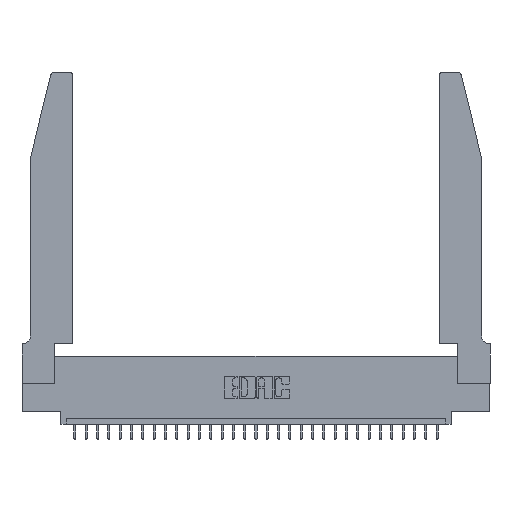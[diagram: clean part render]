
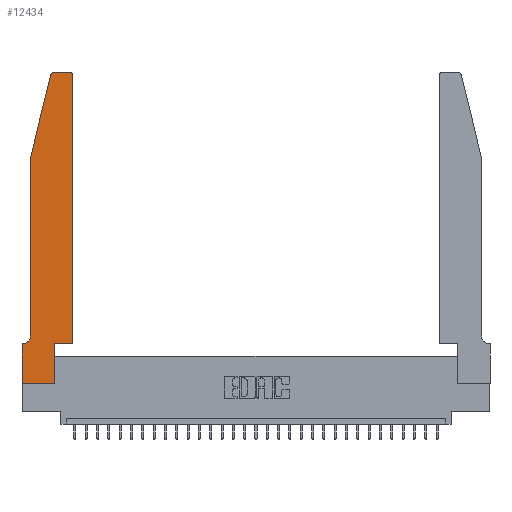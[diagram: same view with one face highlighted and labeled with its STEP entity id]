
A CAD part, top view. The second image highlights one B-rep face of the part: STEP entity #12434.
In plain terms, the highlighted planar face has unit normal (0, 0, 1).
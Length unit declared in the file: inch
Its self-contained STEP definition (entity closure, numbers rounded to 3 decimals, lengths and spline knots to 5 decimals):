
#24 = CARTESIAN_POINT ( 'NONE',  ( 0.4505, 0.35, 0.37 ) ) ;
#184 = DIRECTION ( 'NONE',  ( 0., 1., 0. ) ) ;
#619 = DIRECTION ( 'NONE',  ( -1., 0., 0. ) ) ;
#630 = VERTEX_POINT ( 'NONE', #18062 ) ;
#817 = LINE ( 'NONE', #17613, #28655 ) ;
#1134 = DIRECTION ( 'NONE',  ( 1., 0., 0. ) ) ;
#1655 = DIRECTION ( 'NONE',  ( -0.239, -0.971, 0. ) ) ;
#1787 = ORIENTED_EDGE ( 'NONE', *, *, #20117, .T. ) ;
#1981 = AXIS2_PLACEMENT_3D ( 'NONE', #28719, #7492, #7812 ) ;
#2095 = ORIENTED_EDGE ( 'NONE', *, *, #12523, .T. ) ;
#2313 = CARTESIAN_POINT ( 'NONE',  ( 0., 0., 0.37 ) ) ;
#2774 = CIRCLE ( 'NONE', #6782, 0.03 ) ;
#2963 = DIRECTION ( 'NONE',  ( 0., -1., 0. ) ) ;
#3488 = VERTEX_POINT ( 'NONE', #30178 ) ;
#3689 = EDGE_CURVE ( 'NONE', #6825, #12220, #12042, .T. ) ;
#4050 = EDGE_CURVE ( 'NONE', #20347, #630, #19760, .T. ) ;
#4278 = DIRECTION ( 'NONE',  ( 0., 0., -1. ) ) ;
#4942 = VERTEX_POINT ( 'NONE', #12701 ) ;
#6218 = AXIS2_PLACEMENT_3D ( 'NONE', #19846, #10734, #8375 ) ;
#6300 = ORIENTED_EDGE ( 'NONE', *, *, #28760, .T. ) ;
#6625 = CARTESIAN_POINT ( 'NONE',  ( 0.0055, 0.35, 0.37 ) ) ;
#6782 = AXIS2_PLACEMENT_3D ( 'NONE', #7217, #21823, #21666 ) ;
#6825 = VERTEX_POINT ( 'NONE', #28835 ) ;
#7217 = CARTESIAN_POINT ( 'NONE',  ( 0.4205, 2.72, 0.37 ) ) ;
#7363 = ORIENTED_EDGE ( 'NONE', *, *, #13226, .T. ) ;
#7492 = DIRECTION ( 'NONE',  ( 0., 0., 1. ) ) ;
#7812 = DIRECTION ( 'NONE',  ( 1., 0., 0. ) ) ;
#8301 = LINE ( 'NONE', #17561, #20855 ) ;
#8375 = DIRECTION ( 'NONE',  ( 1., 0., 0. ) ) ;
#9555 = FACE_OUTER_BOUND ( 'NONE', #12694, .T. ) ;
#9701 = ORIENTED_EDGE ( 'NONE', *, *, #3689, .T. ) ;
#10126 = LINE ( 'NONE', #10582, #14154 ) ;
#10496 = CARTESIAN_POINT ( 'NONE',  ( 0.0755, 0.35, 0.37 ) ) ;
#10582 = CARTESIAN_POINT ( 'NONE',  ( 0.2605, 2.75, 0.37 ) ) ;
#10734 = DIRECTION ( 'NONE',  ( 0., 0., 1. ) ) ;
#11142 = VERTEX_POINT ( 'NONE', #6625 ) ;
#11200 = CARTESIAN_POINT ( 'NONE',  ( 0.0055, 0.42, 0.37 ) ) ;
#12042 = LINE ( 'NONE', #2313, #20782 ) ;
#12220 = VERTEX_POINT ( 'NONE', #27486 ) ;
#12434 = ADVANCED_FACE ( 'NONE', ( #9555 ), #19130, .T. ) ;
#12523 = EDGE_CURVE ( 'NONE', #12220, #22360, #26992, .T. ) ;
#12694 = EDGE_LOOP ( 'NONE', ( #1787, #26218, #27043, #19061, #6300, #14378, #14070, #9701, #2095, #24430, #7363, #16059 ) ) ;
#12701 = CARTESIAN_POINT ( 'NONE',  ( 0.4505, 2.72, 0.37 ) ) ;
#12986 = VECTOR ( 'NONE', #1655, 39.37008 ) ;
#13226 = EDGE_CURVE ( 'NONE', #3488, #4942, #14142, .T. ) ;
#13832 = VERTEX_POINT ( 'NONE', #27920 ) ;
#14070 = ORIENTED_EDGE ( 'NONE', *, *, #25275, .T. ) ;
#14142 = LINE ( 'NONE', #24, #26100 ) ;
#14154 = VECTOR ( 'NONE', #29294, 39.37008 ) ;
#14342 = EDGE_CURVE ( 'NONE', #630, #13832, #19048, .T. ) ;
#14378 = ORIENTED_EDGE ( 'NONE', *, *, #29423, .T. ) ;
#14884 = DIRECTION ( 'NONE',  ( 0., 1., 0. ) ) ;
#15767 = VERTEX_POINT ( 'NONE', #30787 ) ;
#15843 = CARTESIAN_POINT ( 'NONE',  ( 0.0755, 2., 0.37 ) ) ;
#16059 = ORIENTED_EDGE ( 'NONE', *, *, #25061, .T. ) ;
#16525 = CARTESIAN_POINT ( 'NONE',  ( 0.0755, 2., 0.37 ) ) ;
#16922 = CARTESIAN_POINT ( 'NONE',  ( 0.2865, 0.35, 0.37 ) ) ;
#17038 = VECTOR ( 'NONE', #14884, 39.37008 ) ;
#17561 = CARTESIAN_POINT ( 'NONE',  ( 0., 0., 0.37 ) ) ;
#17613 = CARTESIAN_POINT ( 'NONE',  ( 0.4505, 0.35, 0.37 ) ) ;
#18062 = CARTESIAN_POINT ( 'NONE',  ( 0.25487, 2.72718, 0.37 ) ) ;
#18419 = DIRECTION ( 'NONE',  ( -1., 0., 0. ) ) ;
#18483 = EDGE_CURVE ( 'NONE', #22360, #3488, #817, .T. ) ;
#19048 = LINE ( 'NONE', #16525, #12986 ) ;
#19061 = ORIENTED_EDGE ( 'NONE', *, *, #29524, .T. ) ;
#19130 = PLANE ( 'NONE',  #1981 ) ;
#19277 = DIRECTION ( 'NONE',  ( 1., 0., 0. ) ) ;
#19760 = CIRCLE ( 'NONE', #6218, 0.03 ) ;
#19846 = CARTESIAN_POINT ( 'NONE',  ( 0.284, 2.72, 0.37 ) ) ;
#20117 = EDGE_CURVE ( 'NONE', #29048, #20347, #10126, .T. ) ;
#20347 = VERTEX_POINT ( 'NONE', #26129 ) ;
#20603 = VECTOR ( 'NONE', #22918, 39.37008 ) ;
#20782 = VECTOR ( 'NONE', #19277, 39.37008 ) ;
#20855 = VECTOR ( 'NONE', #2963, 39.37008 ) ;
#21666 = DIRECTION ( 'NONE',  ( 1., 0., 0. ) ) ;
#21823 = DIRECTION ( 'NONE',  ( 0., 0., 1. ) ) ;
#22360 = VERTEX_POINT ( 'NONE', #26810 ) ;
#22918 = DIRECTION ( 'NONE',  ( 0., -1., 0. ) ) ;
#24430 = ORIENTED_EDGE ( 'NONE', *, *, #18483, .T. ) ;
#24562 = AXIS2_PLACEMENT_3D ( 'NONE', #11200, #4278, #18419 ) ;
#24852 = CARTESIAN_POINT ( 'NONE',  ( 0.4205, 2.75, 0.37 ) ) ;
#25061 = EDGE_CURVE ( 'NONE', #4942, #29048, #2774, .T. ) ;
#25275 = EDGE_CURVE ( 'NONE', #15767, #6825, #8301, .T. ) ;
#25448 = CARTESIAN_POINT ( 'NONE',  ( 0.0755, 0.42, 0.37 ) ) ;
#26100 = VECTOR ( 'NONE', #184, 39.37008 ) ;
#26129 = CARTESIAN_POINT ( 'NONE',  ( 0.284, 2.75, 0.37 ) ) ;
#26218 = ORIENTED_EDGE ( 'NONE', *, *, #4050, .T. ) ;
#26810 = CARTESIAN_POINT ( 'NONE',  ( 0.2865, 0.35, 0.37 ) ) ;
#26992 = LINE ( 'NONE', #16922, #17038 ) ;
#27043 = ORIENTED_EDGE ( 'NONE', *, *, #14342, .T. ) ;
#27320 = LINE ( 'NONE', #10496, #30609 ) ;
#27486 = CARTESIAN_POINT ( 'NONE',  ( 0.2865, 0., 0.37 ) ) ;
#27920 = CARTESIAN_POINT ( 'NONE',  ( 0.0755, 2., 0.37 ) ) ;
#28091 = LINE ( 'NONE', #15843, #20603 ) ;
#28655 = VECTOR ( 'NONE', #1134, 39.37008 ) ;
#28719 = CARTESIAN_POINT ( 'NONE',  ( 0., 0.35, 0.37 ) ) ;
#28760 = EDGE_CURVE ( 'NONE', #30773, #11142, #30079, .T. ) ;
#28835 = CARTESIAN_POINT ( 'NONE',  ( 0., 0., 0.37 ) ) ;
#29048 = VERTEX_POINT ( 'NONE', #24852 ) ;
#29294 = DIRECTION ( 'NONE',  ( -1., 0., 0. ) ) ;
#29423 = EDGE_CURVE ( 'NONE', #11142, #15767, #27320, .T. ) ;
#29524 = EDGE_CURVE ( 'NONE', #13832, #30773, #28091, .T. ) ;
#30079 = CIRCLE ( 'NONE', #24562, 0.07 ) ;
#30178 = CARTESIAN_POINT ( 'NONE',  ( 0.4505, 0.35, 0.37 ) ) ;
#30609 = VECTOR ( 'NONE', #619, 39.37008 ) ;
#30773 = VERTEX_POINT ( 'NONE', #25448 ) ;
#30787 = CARTESIAN_POINT ( 'NONE',  ( 0., 0.35, 0.37 ) ) ;
